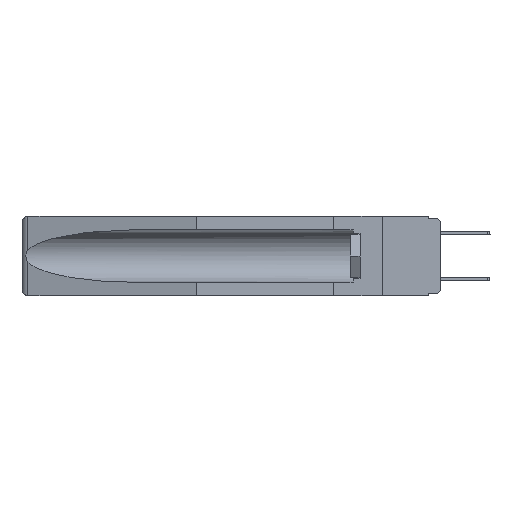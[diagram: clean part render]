
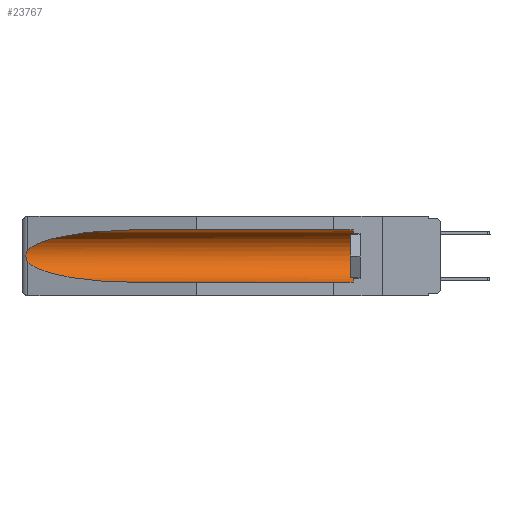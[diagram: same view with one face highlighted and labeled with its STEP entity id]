
A CAD part, left-side view. The second image highlights one B-rep face of the part: STEP entity #23767.
In plain terms, the highlighted cylindrical face has radius 2.857 mm (diameter 5.715 mm), a partial arc.
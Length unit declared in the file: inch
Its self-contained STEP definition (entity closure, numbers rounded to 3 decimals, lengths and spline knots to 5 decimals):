
#9 = CARTESIAN_POINT ( 'NONE',  ( 0.155, -0.30754, -0.284 ) ) ;
#635 = CARTESIAN_POINT ( 'NONE',  ( 0.2673, 1.5327, -0.16383 ) ) ;
#764 = CARTESIAN_POINT ( 'NONE',  ( 0.26655, 1.53094, -0.18657 ) ) ;
#4013 = EDGE_CURVE ( 'NONE', #21104, #22125, #11843, .T. ) ;
#4530 = ORIENTED_EDGE ( 'NONE', *, *, #4013, .T. ) ;
#5011 = CYLINDRICAL_SURFACE ( 'NONE', #22991, 0.1125 ) ;
#5086 = VECTOR ( 'NONE', #15578, 39.37008 ) ;
#5127 = CARTESIAN_POINT ( 'NONE',  ( 0.21114, 1.30732, -0.284 ) ) ;
#5370 = DIRECTION ( 'NONE',  ( 0., 0., 1. ) ) ;
#6238 = CARTESIAN_POINT ( 'NONE',  ( 0.2675, 1.53308, -0.16763 ) ) ;
#6317 = AXIS2_PLACEMENT_3D ( 'NONE', #21020, #8674, #14553 ) ;
#6892 = CARTESIAN_POINT ( 'NONE',  ( 0.25451, 1.48313, -0.09465 ) ) ;
#6996 = VERTEX_POINT ( 'NONE', #20786 ) ;
#7326 = ORIENTED_EDGE ( 'NONE', *, *, #24005, .F. ) ;
#7436 = CARTESIAN_POINT ( 'NONE',  ( 0.155, -0.30754, -0.059 ) ) ;
#7629 = ORIENTED_EDGE ( 'NONE', *, *, #22223, .T. ) ;
#8411 = CARTESIAN_POINT ( 'NONE',  ( 0.26597, 1.52961, -0.15275 ) ) ;
#8583 = CARTESIAN_POINT ( 'NONE',  ( 0.26537, 1.52718, -0.19328 ) ) ;
#8674 = DIRECTION ( 'NONE',  ( 0., -1., 0. ) ) ;
#9217 = CARTESIAN_POINT ( 'NONE',  ( 0.155, -0.30754, -0.1715 ) ) ;
#9311 = EDGE_CURVE ( 'NONE', #24988, #6996, #13295, .T. ) ;
#9344 = DIRECTION ( 'NONE',  ( 0., 1., 0. ) ) ;
#9481 = VERTEX_POINT ( 'NONE', #24372 ) ;
#10185 = ORIENTED_EDGE ( 'NONE', *, *, #9311, .T. ) ;
#11843 = B_SPLINE_CURVE_WITH_KNOTS ( 'NONE', 3,
 ( #23851, #8411, #19643, #635, #6238, #14288, #12356, #764, #21688, #12110 ),
 .UNSPECIFIED., .F., .F.,
 ( 4, 2, 2, 2, 4 ),
 ( 0., 0.00029, 0.00058, 0.00087, 0.00117 ),
 .UNSPECIFIED. ) ;
#12110 = CARTESIAN_POINT ( 'NONE',  ( 0.26537, 1.52718, -0.19328 ) ) ;
#12208 = CARTESIAN_POINT ( 'NONE',  ( 0.26537, 1.52718, -0.14972 ) ) ;
#12356 = CARTESIAN_POINT ( 'NONE',  ( 0.2673, 1.53269, -0.17917 ) ) ;
#13212 = CARTESIAN_POINT ( 'NONE',  ( 0.155, 1.07973, -0.059 ) ) ;
#13295 = LINE ( 'NONE', #7436, #22742 ) ;
#13521 = ORIENTED_EDGE ( 'NONE', *, *, #22842, .T. ) ;
#13830 = EDGE_LOOP ( 'NONE', ( #18929, #4530, #7629, #7326, #13521, #10185 ) ) ;
#14058 = CIRCLE ( 'NONE', #6317, 0.1125 ) ;
#14288 = CARTESIAN_POINT ( 'NONE',  ( 0.2675, 1.53308, -0.17534 ) ) ;
#14447 = CARTESIAN_POINT ( 'NONE',  ( 0.25451, 1.48313, -0.24835 ) ) ;
#14519 =( BOUNDED_CURVE ( )  B_SPLINE_CURVE ( 3, ( #8583, #14447, #5127, #24649 ),
 .UNSPECIFIED., .F., .T. ) 
 B_SPLINE_CURVE_WITH_KNOTS ( ( 4, 4 ),
 ( 0.1948, 1.5708 ),
 .UNSPECIFIED. ) 
 CURVE ( )  GEOMETRIC_REPRESENTATION_ITEM ( )  RATIONAL_B_SPLINE_CURVE ( ( 1., 0.848, 0.848, 1. ) ) 
 REPRESENTATION_ITEM ( '' )  );
#14553 = DIRECTION ( 'NONE',  ( 0., 0., 1. ) ) ;
#14667 =( BOUNDED_CURVE ( )  B_SPLINE_CURVE ( 3, ( #13212, #17182, #6892, #14675 ),
 .UNSPECIFIED., .F., .T. ) 
 B_SPLINE_CURVE_WITH_KNOTS ( ( 4, 4 ),
 ( 4.71239, 6.08839 ),
 .UNSPECIFIED. ) 
 CURVE ( )  GEOMETRIC_REPRESENTATION_ITEM ( )  RATIONAL_B_SPLINE_CURVE ( ( 1., 0.848, 0.848, 1. ) ) 
 REPRESENTATION_ITEM ( '' )  );
#14675 = CARTESIAN_POINT ( 'NONE',  ( 0.26537, 1.52718, -0.14972 ) ) ;
#15217 = DIRECTION ( 'NONE',  ( 0., 1., 0. ) ) ;
#15578 = DIRECTION ( 'NONE',  ( 0., 1., 0. ) ) ;
#16369 = CARTESIAN_POINT ( 'NONE',  ( 0.155, 0.126, -0.059 ) ) ;
#17182 = CARTESIAN_POINT ( 'NONE',  ( 0.21114, 1.30732, -0.059 ) ) ;
#17496 = LINE ( 'NONE', #9, #5086 ) ;
#18929 = ORIENTED_EDGE ( 'NONE', *, *, #22890, .T. ) ;
#19643 = CARTESIAN_POINT ( 'NONE',  ( 0.26654, 1.53092, -0.15636 ) ) ;
#19987 = CARTESIAN_POINT ( 'NONE',  ( 0.155, 0.126, -0.284 ) ) ;
#20707 = CARTESIAN_POINT ( 'NONE',  ( 0.26537, 1.52718, -0.19328 ) ) ;
#20786 = CARTESIAN_POINT ( 'NONE',  ( 0.155, 1.07973, -0.059 ) ) ;
#21020 = CARTESIAN_POINT ( 'NONE',  ( 0.155, 0.126, -0.1715 ) ) ;
#21104 = VERTEX_POINT ( 'NONE', #12208 ) ;
#21688 = CARTESIAN_POINT ( 'NONE',  ( 0.26597, 1.5296, -0.19026 ) ) ;
#22125 = VERTEX_POINT ( 'NONE', #20707 ) ;
#22223 = EDGE_CURVE ( 'NONE', #22125, #9481, #14519, .T. ) ;
#22742 = VECTOR ( 'NONE', #15217, 39.37008 ) ;
#22842 = EDGE_CURVE ( 'NONE', #23237, #24988, #14058, .T. ) ;
#22890 = EDGE_CURVE ( 'NONE', #6996, #21104, #14667, .T. ) ;
#22991 = AXIS2_PLACEMENT_3D ( 'NONE', #9217, #9344, #5370 ) ;
#23237 = VERTEX_POINT ( 'NONE', #19987 ) ;
#23767 = ADVANCED_FACE ( 'NONE', ( #24533 ), #5011, .F. ) ;
#23851 = CARTESIAN_POINT ( 'NONE',  ( 0.26537, 1.52718, -0.14972 ) ) ;
#24005 = EDGE_CURVE ( 'NONE', #23237, #9481, #17496, .T. ) ;
#24372 = CARTESIAN_POINT ( 'NONE',  ( 0.155, 1.07973, -0.284 ) ) ;
#24533 = FACE_OUTER_BOUND ( 'NONE', #13830, .T. ) ;
#24649 = CARTESIAN_POINT ( 'NONE',  ( 0.155, 1.07973, -0.284 ) ) ;
#24988 = VERTEX_POINT ( 'NONE', #16369 ) ;
